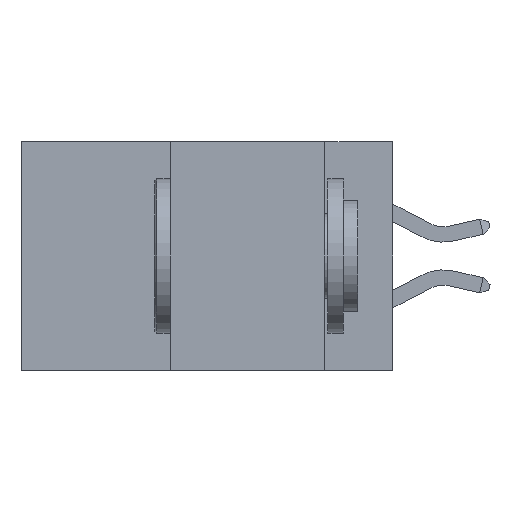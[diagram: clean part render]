
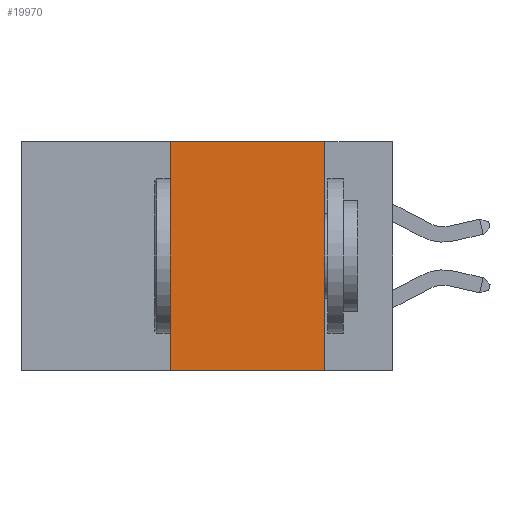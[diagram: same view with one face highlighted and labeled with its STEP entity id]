
A CAD part, left-side view. The second image highlights one B-rep face of the part: STEP entity #19970.
In plain terms, the highlighted planar face has unit normal (-1, 0, 0).
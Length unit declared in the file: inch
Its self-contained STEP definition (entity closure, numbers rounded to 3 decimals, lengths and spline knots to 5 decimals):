
#268 = VERTEX_POINT ( 'NONE', #7644 ) ;
#514 = CARTESIAN_POINT ( 'NONE',  ( 0., 0.11, 0. ) ) ;
#946 = CARTESIAN_POINT ( 'NONE',  ( 0., 0.6, 0. ) ) ;
#1032 = CARTESIAN_POINT ( 'NONE',  ( 0., 0.6, 0. ) ) ;
#1438 = EDGE_CURVE ( 'NONE', #27749, #5894, #2668, .T. ) ;
#1657 = DIRECTION ( 'NONE',  ( 0., 0., 1. ) ) ;
#2668 = LINE ( 'NONE', #946, #18347 ) ;
#2836 = EDGE_CURVE ( 'NONE', #5894, #26172, #17572, .T. ) ;
#2854 = LINE ( 'NONE', #10495, #25129 ) ;
#3599 = AXIS2_PLACEMENT_3D ( 'NONE', #1032, #12315, #21271 ) ;
#5894 = VERTEX_POINT ( 'NONE', #514 ) ;
#6001 = ORIENTED_EDGE ( 'NONE', *, *, #1438, .F. ) ;
#7644 = CARTESIAN_POINT ( 'NONE',  ( 0., 0.36, -0.37 ) ) ;
#7811 = DIRECTION ( 'NONE',  ( 0., -1., 0. ) ) ;
#7837 = ORIENTED_EDGE ( 'NONE', *, *, #10491, .T. ) ;
#9498 = VECTOR ( 'NONE', #26510, 39.37008 ) ;
#10491 = EDGE_CURVE ( 'NONE', #268, #26172, #14261, .T. ) ;
#10495 = CARTESIAN_POINT ( 'NONE',  ( 0., 0.36, 0. ) ) ;
#11701 = ORIENTED_EDGE ( 'NONE', *, *, #2836, .F. ) ;
#12315 = DIRECTION ( 'NONE',  ( 1., 0., 0. ) ) ;
#14261 = LINE ( 'NONE', #15008, #17778 ) ;
#15008 = CARTESIAN_POINT ( 'NONE',  ( 0., 0.6, -0.37 ) ) ;
#16753 = ORIENTED_EDGE ( 'NONE', *, *, #21830, .F. ) ;
#17262 = DIRECTION ( 'NONE',  ( 0., -1., 0. ) ) ;
#17430 = CARTESIAN_POINT ( 'NONE',  ( 0., 0.11, 0. ) ) ;
#17572 = LINE ( 'NONE', #17430, #9498 ) ;
#17778 = VECTOR ( 'NONE', #17262, 39.37008 ) ;
#18347 = VECTOR ( 'NONE', #7811, 39.37008 ) ;
#18403 = CARTESIAN_POINT ( 'NONE',  ( 0., 0.36, 0. ) ) ;
#19238 = PLANE ( 'NONE',  #3599 ) ;
#19970 = ADVANCED_FACE ( 'NONE', ( #28009 ), #19238, .F. ) ;
#21271 = DIRECTION ( 'NONE',  ( 0., 0., -1. ) ) ;
#21830 = EDGE_CURVE ( 'NONE', #268, #27749, #2854, .T. ) ;
#22197 = EDGE_LOOP ( 'NONE', ( #11701, #6001, #16753, #7837 ) ) ;
#25129 = VECTOR ( 'NONE', #1657, 39.37008 ) ;
#26172 = VERTEX_POINT ( 'NONE', #26413 ) ;
#26413 = CARTESIAN_POINT ( 'NONE',  ( 0., 0.11, -0.37 ) ) ;
#26510 = DIRECTION ( 'NONE',  ( 0., 0., -1. ) ) ;
#27749 = VERTEX_POINT ( 'NONE', #18403 ) ;
#28009 = FACE_OUTER_BOUND ( 'NONE', #22197, .T. ) ;
